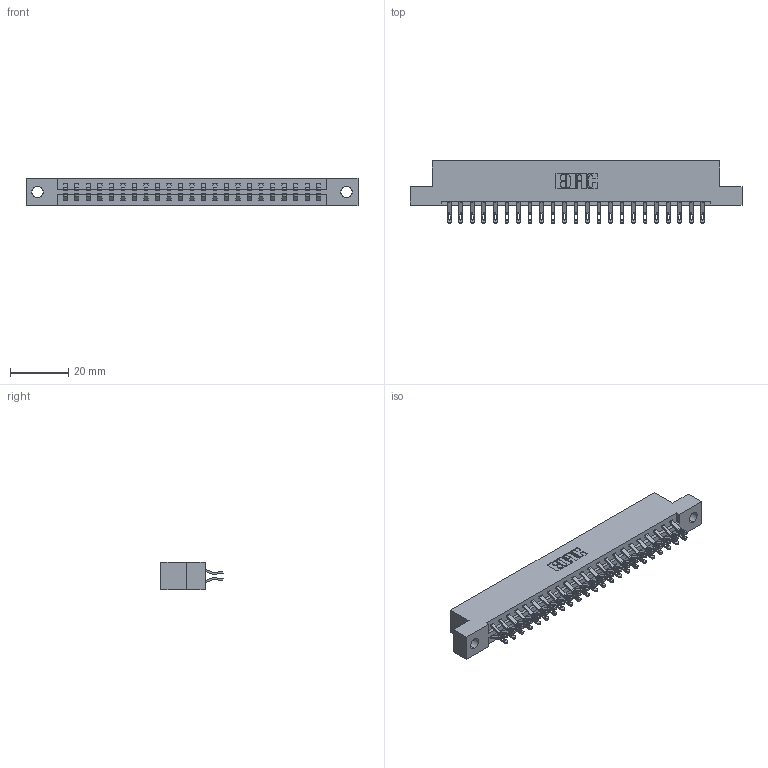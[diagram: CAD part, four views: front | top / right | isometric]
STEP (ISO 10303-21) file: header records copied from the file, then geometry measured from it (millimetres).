
FILE_DESCRIPTION (( 'STEP AP203' ), '1' );
FILE_NAME ('387-046-555-204.STEP', '2019-10-18T08:06:52', ( '' ), ( '' ), 'SwSTEP 2.0', 'SolidWorks 2016', '' );
FILE_SCHEMA (( 'CONFIG_CONTROL_DESIGN' ));
Length unit declared in the file: inch
Products named in the file (3): 345-292-001_555 Tail; 387-046-555-204; 337 Part_Flush Mounting Lugs - 0.156 Dia-TH
Assembly tree (47 placements, depth 2):
  387-046-555-204
    337 Part_Flush Mounting Lugs - 0.156 Dia-TH
    345-292-001_555 Tail  x46
Bounding box: 114.15 x 21.47 x 9.4 mm (x, y, z)
Volume: 11822.4 mm3; surface area: 13480.9 mm2
Topology: 47 solids, 47 shells, 2874 faces, 9005 edges, 6002 vertices
Faces by surface type: plane 1726, cylinder 1148
Entity records: 20619 total; most frequent: CARTESIAN_POINT 3524, ORIENTED_EDGE 3430, DIRECTION 3003, EDGE_CURVE 1715, VECTOR 1567, LINE 1567, VERTEX_POINT 1142, AXIS2_PLACEMENT_3D 718
